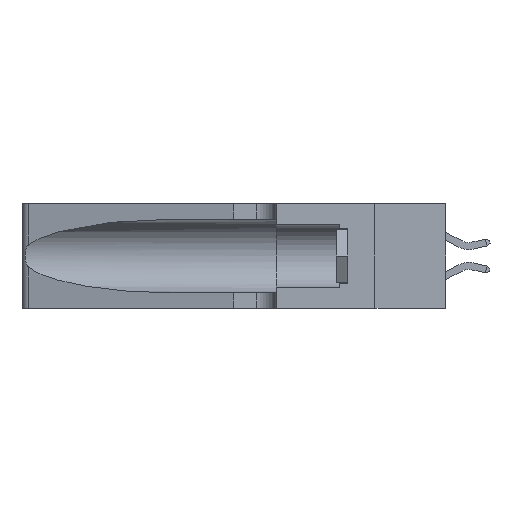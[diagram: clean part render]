
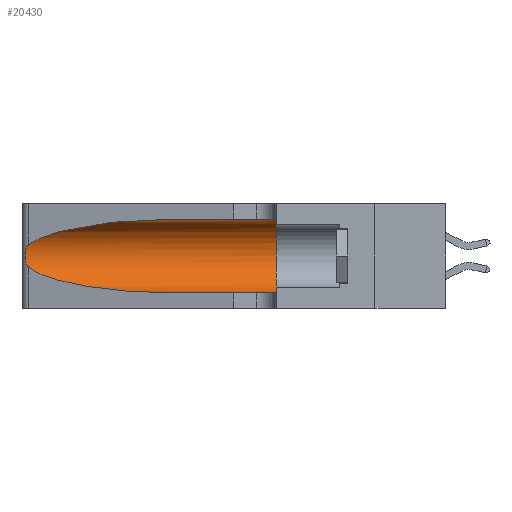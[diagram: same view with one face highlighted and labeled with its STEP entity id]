
A CAD part, left-side view. The second image highlights one B-rep face of the part: STEP entity #20430.
In plain terms, the highlighted cylindrical face has radius 3.308 mm (diameter 6.617 mm), a partial arc.
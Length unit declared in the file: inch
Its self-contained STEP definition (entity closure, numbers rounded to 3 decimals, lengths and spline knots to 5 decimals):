
#548 = CARTESIAN_POINT ( 'NONE',  ( 0.25555, 1.22994, 0.2215 ) ) ;
#2233 = EDGE_CURVE ( 'NONE', #6101, #7218, #34051, .T. ) ;
#2985 = CARTESIAN_POINT ( 'NONE',  ( 0.1305, 1.61858, 0.185 ) ) ;
#3008 = CARTESIAN_POINT ( 'NONE',  ( 0.1305, 0.35, 0.31525 ) ) ;
#3431 = CARTESIAN_POINT ( 'NONE',  ( 0.25787, 1.23484, 0.2124 ) ) ;
#3555 = CARTESIAN_POINT ( 'NONE',  ( 0.25487, 1.22718, 0.22369 ) ) ;
#3970 = CARTESIAN_POINT ( 'NONE',  ( 0.1305, 0.72297, 0.31525 ) ) ;
#4033 = VERTEX_POINT ( 'NONE', #22077 ) ;
#5319 = CARTESIAN_POINT ( 'NONE',  ( 0.1305, 0.35, 0.05475 ) ) ;
#6101 = VERTEX_POINT ( 'NONE', #3008 ) ;
#6294 = CARTESIAN_POINT ( 'NONE',  ( 0.26018, 1.23835, 0.19895 ) ) ;
#6677 = CARTESIAN_POINT ( 'NONE',  ( 0.1305, 0.72297, 0.05475 ) ) ;
#6899 = EDGE_CURVE ( 'NONE', #31584, #4033, #21336, .T. ) ;
#7218 = VERTEX_POINT ( 'NONE', #5319 ) ;
#7781 = VECTOR ( 'NONE', #10788, 39.37008 ) ;
#8638 = CARTESIAN_POINT ( 'NONE',  ( 0.1305, 0.72297, 0.31525 ) ) ;
#8935 = DIRECTION ( 'NONE',  ( 0., 1., 0. ) ) ;
#9153 = CARTESIAN_POINT ( 'NONE',  ( 0.26075, 1.23896, 0.178 ) ) ;
#10788 = DIRECTION ( 'NONE',  ( 0., -1., 0. ) ) ;
#11326 = VERTEX_POINT ( 'NONE', #3555 ) ;
#11492 = AXIS2_PLACEMENT_3D ( 'NONE', #2985, #28031, #33578 ) ;
#11567 = CYLINDRICAL_SURFACE ( 'NONE', #11492, 0.13025 ) ;
#11985 = CARTESIAN_POINT ( 'NONE',  ( 0.25856, 1.23593, 0.16098 ) ) ;
#13839 = ORIENTED_EDGE ( 'NONE', *, *, #18141, .T. ) ;
#14766 = CARTESIAN_POINT ( 'NONE',  ( 0.25639, 1.23186, 0.15144 ) ) ;
#15398 = VERTEX_POINT ( 'NONE', #3970 ) ;
#16257 = ORIENTED_EDGE ( 'NONE', *, *, #31144, .T. ) ;
#17046 = CARTESIAN_POINT ( 'NONE',  ( 0.25487, 1.22718, 0.22369 ) ) ;
#17419 = CARTESIAN_POINT ( 'NONE',  ( 0.25487, 1.22718, 0.22369 ) ) ;
#17534 = CARTESIAN_POINT ( 'NONE',  ( 0.25487, 1.22718, 0.14631 ) ) ;
#17807 = CARTESIAN_POINT ( 'NONE',  ( 0.2373, 1.15595, 0.08982 ) ) ;
#17862 = DIRECTION ( 'NONE',  ( 0., -1., 0. ) ) ;
#17920 = ORIENTED_EDGE ( 'NONE', *, *, #6899, .T. ) ;
#18141 = EDGE_CURVE ( 'NONE', #15398, #11326, #26202, .T. ) ;
#20245 = CARTESIAN_POINT ( 'NONE',  ( 0.25639, 1.23184, 0.21858 ) ) ;
#20430 = ADVANCED_FACE ( 'NONE', ( #26247 ), #11567, .F. ) ;
#20621 = CARTESIAN_POINT ( 'NONE',  ( 0.25487, 1.22718, 0.14631 ) ) ;
#21336 =( BOUNDED_CURVE ( )  B_SPLINE_CURVE ( 3, ( #20621, #17807, #23357, #6677 ),
 .UNSPECIFIED., .F., .F. ) 
 B_SPLINE_CURVE_WITH_KNOTS ( ( 4, 4 ),
 ( 3.44316, 4.71239 ),
 .UNSPECIFIED. ) 
 CURVE ( )  GEOMETRIC_REPRESENTATION_ITEM ( )  RATIONAL_B_SPLINE_CURVE ( ( 1., 0.87, 0.87, 1. ) ) 
 REPRESENTATION_ITEM ( '' )  );
#22008 = EDGE_CURVE ( 'NONE', #15398, #6101, #33477, .T. ) ;
#22077 = CARTESIAN_POINT ( 'NONE',  ( 0.1305, 0.72297, 0.05475 ) ) ;
#22118 = ORIENTED_EDGE ( 'NONE', *, *, #33199, .T. ) ;
#22129 = CARTESIAN_POINT ( 'NONE',  ( 0.25487, 1.22718, 0.14631 ) ) ;
#22826 = B_SPLINE_CURVE_WITH_KNOTS ( 'NONE', 3,
 ( #17419, #548, #20245, #3431, #22961, #6294, #25719, #9153, #28453, #11985, #31215, #14766, #33999, #17534 ),
 .UNSPECIFIED., .F., .F.,
 ( 4, 2, 2, 2, 2, 2, 4 ),
 ( 0., 0.00027, 0.00053, 0.00107, 0.0016, 0.00187, 0.00214 ),
 .UNSPECIFIED. ) ;
#22961 = CARTESIAN_POINT ( 'NONE',  ( 0.25854, 1.2359, 0.20912 ) ) ;
#23357 = CARTESIAN_POINT ( 'NONE',  ( 0.18966, 0.96281, 0.05475 ) ) ;
#23443 = LINE ( 'NONE', #24663, #7781 ) ;
#23794 = ORIENTED_EDGE ( 'NONE', *, *, #2233, .F. ) ;
#24663 = CARTESIAN_POINT ( 'NONE',  ( 0.1305, 1.61858, 0.05475 ) ) ;
#25509 = CARTESIAN_POINT ( 'NONE',  ( 0.1305, 0.35, 0.185 ) ) ;
#25719 = CARTESIAN_POINT ( 'NONE',  ( 0.26075, 1.23896, 0.19203 ) ) ;
#26182 = VECTOR ( 'NONE', #17862, 39.37008 ) ;
#26202 =( BOUNDED_CURVE ( )  B_SPLINE_CURVE ( 3, ( #8638, #30714, #33501, #17046 ),
 .UNSPECIFIED., .F., .T. ) 
 B_SPLINE_CURVE_WITH_KNOTS ( ( 4, 4 ),
 ( 1.5708, 2.84003 ),
 .UNSPECIFIED. ) 
 CURVE ( )  GEOMETRIC_REPRESENTATION_ITEM ( )  RATIONAL_B_SPLINE_CURVE ( ( 1., 0.87, 0.87, 1. ) ) 
 REPRESENTATION_ITEM ( '' )  );
#26247 = FACE_OUTER_BOUND ( 'NONE', #33350, .T. ) ;
#28031 = DIRECTION ( 'NONE',  ( 0., -1., 0. ) ) ;
#28249 = DIRECTION ( 'NONE',  ( 0., 0., 1. ) ) ;
#28453 = CARTESIAN_POINT ( 'NONE',  ( 0.26017, 1.23833, 0.17102 ) ) ;
#29590 = ORIENTED_EDGE ( 'NONE', *, *, #22008, .F. ) ;
#30714 = CARTESIAN_POINT ( 'NONE',  ( 0.18966, 0.96281, 0.31525 ) ) ;
#31144 = EDGE_CURVE ( 'NONE', #11326, #31584, #22826, .T. ) ;
#31215 = CARTESIAN_POINT ( 'NONE',  ( 0.25789, 1.23486, 0.15765 ) ) ;
#31584 = VERTEX_POINT ( 'NONE', #22129 ) ;
#32430 = AXIS2_PLACEMENT_3D ( 'NONE', #25509, #8935, #28249 ) ;
#33199 = EDGE_CURVE ( 'NONE', #4033, #7218, #23443, .T. ) ;
#33350 = EDGE_LOOP ( 'NONE', ( #13839, #16257, #17920, #22118, #23794, #29590 ) ) ;
#33477 = LINE ( 'NONE', #34323, #26182 ) ;
#33501 = CARTESIAN_POINT ( 'NONE',  ( 0.2373, 1.15595, 0.28018 ) ) ;
#33578 = DIRECTION ( 'NONE',  ( 0., 0., -1. ) ) ;
#33999 = CARTESIAN_POINT ( 'NONE',  ( 0.25555, 1.22993, 0.14849 ) ) ;
#34051 = CIRCLE ( 'NONE', #32430, 0.13025 ) ;
#34323 = CARTESIAN_POINT ( 'NONE',  ( 0.1305, 1.61858, 0.31525 ) ) ;
